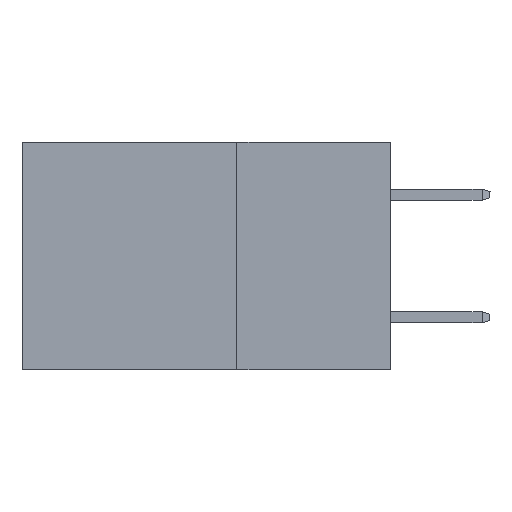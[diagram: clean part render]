
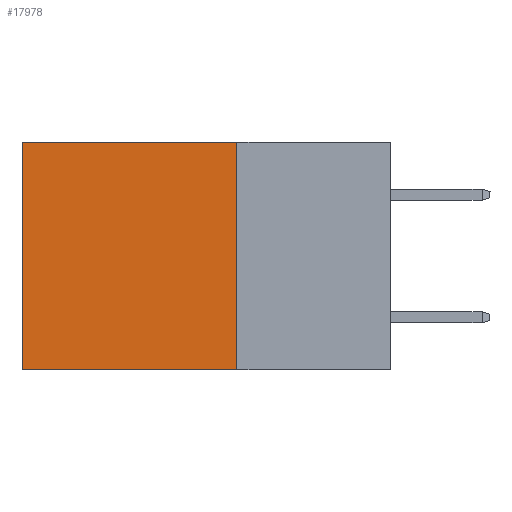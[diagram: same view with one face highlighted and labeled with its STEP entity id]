
A CAD part, left-side view. The second image highlights one B-rep face of the part: STEP entity #17978.
In plain terms, the highlighted planar face has unit normal (-1, 0, 0).
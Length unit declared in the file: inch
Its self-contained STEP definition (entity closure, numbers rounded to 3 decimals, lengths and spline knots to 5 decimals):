
#133 = EDGE_CURVE ( 'NONE', #44955, #2363, #11537, .T. ) ;
#921 = ORIENTED_EDGE ( 'NONE', *, *, #133, .F. ) ;
#2144 = CARTESIAN_POINT ( 'NONE',  ( 0.2875, 0.6, 0. ) ) ;
#2363 = VERTEX_POINT ( 'NONE', #37878 ) ;
#2424 = CARTESIAN_POINT ( 'NONE',  ( 0.2875, 0.6, -0.37 ) ) ;
#3410 = CARTESIAN_POINT ( 'NONE',  ( 0.2875, 0.6, 0. ) ) ;
#7301 = DIRECTION ( 'NONE',  ( 0., 0., -1. ) ) ;
#7423 = VERTEX_POINT ( 'NONE', #2144 ) ;
#8025 = ORIENTED_EDGE ( 'NONE', *, *, #25125, .T. ) ;
#8462 = AXIS2_PLACEMENT_3D ( 'NONE', #36093, #14582, #39620 ) ;
#9231 = LINE ( 'NONE', #43253, #27561 ) ;
#10320 = EDGE_LOOP ( 'NONE', ( #8025, #31393, #921, #18515 ) ) ;
#10846 = PLANE ( 'NONE',  #8462 ) ;
#11378 = VECTOR ( 'NONE', #26463, 39.37008 ) ;
#11537 = LINE ( 'NONE', #19368, #11378 ) ;
#14582 = DIRECTION ( 'NONE',  ( 1., 0., 0. ) ) ;
#17978 = ADVANCED_FACE ( 'NONE', ( #45406 ), #10846, .F. ) ;
#18515 = ORIENTED_EDGE ( 'NONE', *, *, #46113, .T. ) ;
#19368 = CARTESIAN_POINT ( 'NONE',  ( 0.2875, 0.25, 0. ) ) ;
#19524 = VECTOR ( 'NONE', #44990, 39.37008 ) ;
#19580 = LINE ( 'NONE', #41682, #19524 ) ;
#20154 = VERTEX_POINT ( 'NONE', #2424 ) ;
#25125 = EDGE_CURVE ( 'NONE', #7423, #20154, #25291, .T. ) ;
#25188 = VECTOR ( 'NONE', #7301, 39.37008 ) ;
#25291 = LINE ( 'NONE', #3410, #25188 ) ;
#26463 = DIRECTION ( 'NONE',  ( 0., 0., -1. ) ) ;
#27561 = VECTOR ( 'NONE', #46540, 39.37008 ) ;
#31393 = ORIENTED_EDGE ( 'NONE', *, *, #38337, .F. ) ;
#36093 = CARTESIAN_POINT ( 'NONE',  ( 0.2875, 0.25, 0. ) ) ;
#37878 = CARTESIAN_POINT ( 'NONE',  ( 0.2875, 0.25, -0.37 ) ) ;
#38337 = EDGE_CURVE ( 'NONE', #2363, #20154, #19580, .T. ) ;
#39620 = DIRECTION ( 'NONE',  ( 0., 0., -1. ) ) ;
#41682 = CARTESIAN_POINT ( 'NONE',  ( 0.2875, 0.25, -0.37 ) ) ;
#42148 = CARTESIAN_POINT ( 'NONE',  ( 0.2875, 0.25, 0. ) ) ;
#43253 = CARTESIAN_POINT ( 'NONE',  ( 0.2875, 0.25, 0. ) ) ;
#44955 = VERTEX_POINT ( 'NONE', #42148 ) ;
#44990 = DIRECTION ( 'NONE',  ( 0., 1., 0. ) ) ;
#45406 = FACE_OUTER_BOUND ( 'NONE', #10320, .T. ) ;
#46113 = EDGE_CURVE ( 'NONE', #44955, #7423, #9231, .T. ) ;
#46540 = DIRECTION ( 'NONE',  ( 0., 1., 0. ) ) ;
